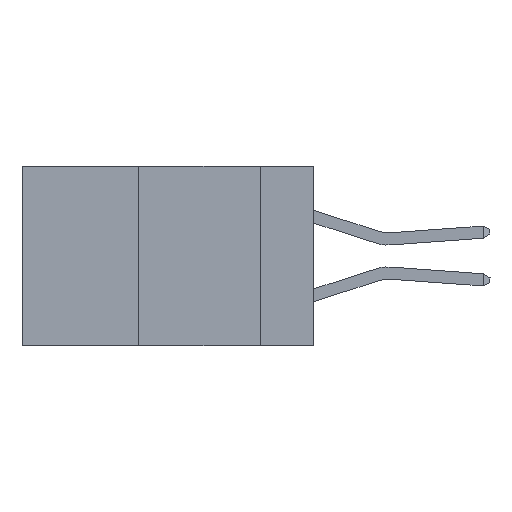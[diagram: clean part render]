
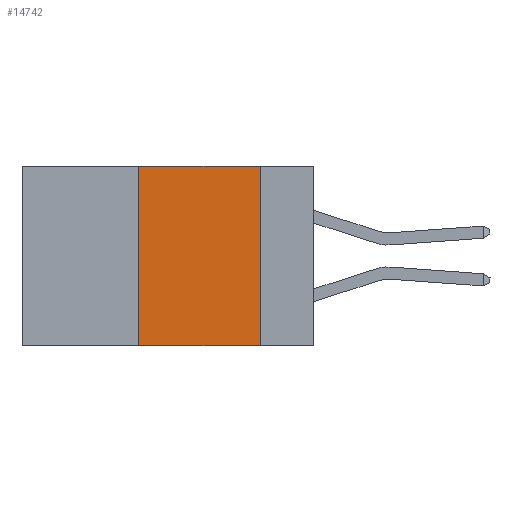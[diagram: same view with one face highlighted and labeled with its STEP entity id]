
A CAD part, left-side view. The second image highlights one B-rep face of the part: STEP entity #14742.
In plain terms, the highlighted planar face has unit normal (-1, 0, 0).
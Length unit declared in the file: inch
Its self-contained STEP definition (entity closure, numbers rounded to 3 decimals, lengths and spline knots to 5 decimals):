
#237 = CARTESIAN_POINT ( 'NONE',  ( 0., 0.11, 0. ) ) ;
#320 = EDGE_CURVE ( 'NONE', #1508, #4824, #4177, .T. ) ;
#327 = PLANE ( 'NONE',  #4135 ) ;
#705 = VECTOR ( 'NONE', #15442, 39.37008 ) ;
#934 = EDGE_CURVE ( 'NONE', #1508, #12777, #6030, .T. ) ;
#1080 = EDGE_CURVE ( 'NONE', #8344, #4824, #12422, .T. ) ;
#1280 = EDGE_CURVE ( 'NONE', #12777, #8344, #11835, .T. ) ;
#1335 = DIRECTION ( 'NONE',  ( 0., -1., 0. ) ) ;
#1414 = CARTESIAN_POINT ( 'NONE',  ( 0., 0.6, 0. ) ) ;
#1508 = VERTEX_POINT ( 'NONE', #4105 ) ;
#1845 = VECTOR ( 'NONE', #1335, 39.37008 ) ;
#3018 = CARTESIAN_POINT ( 'NONE',  ( 0., 0.6, -0.37 ) ) ;
#4105 = CARTESIAN_POINT ( 'NONE',  ( 0., 0.36, -0.37 ) ) ;
#4135 = AXIS2_PLACEMENT_3D ( 'NONE', #11725, #4278, #12941 ) ;
#4177 = LINE ( 'NONE', #3018, #705 ) ;
#4278 = DIRECTION ( 'NONE',  ( 1., 0., 0. ) ) ;
#4783 = ORIENTED_EDGE ( 'NONE', *, *, #934, .F. ) ;
#4824 = VERTEX_POINT ( 'NONE', #6636 ) ;
#5525 = CARTESIAN_POINT ( 'NONE',  ( 0., 0.36, 0. ) ) ;
#6030 = LINE ( 'NONE', #10517, #15502 ) ;
#6633 = FACE_OUTER_BOUND ( 'NONE', #8997, .T. ) ;
#6636 = CARTESIAN_POINT ( 'NONE',  ( 0., 0.11, -0.37 ) ) ;
#8344 = VERTEX_POINT ( 'NONE', #13882 ) ;
#8997 = EDGE_LOOP ( 'NONE', ( #9445, #13893, #4783, #11400 ) ) ;
#9445 = ORIENTED_EDGE ( 'NONE', *, *, #1080, .F. ) ;
#10517 = CARTESIAN_POINT ( 'NONE',  ( 0., 0.36, 0. ) ) ;
#11400 = ORIENTED_EDGE ( 'NONE', *, *, #320, .T. ) ;
#11469 = DIRECTION ( 'NONE',  ( 0., 0., 1. ) ) ;
#11725 = CARTESIAN_POINT ( 'NONE',  ( 0., 0.6, 0. ) ) ;
#11835 = LINE ( 'NONE', #1414, #1845 ) ;
#12422 = LINE ( 'NONE', #237, #16074 ) ;
#12777 = VERTEX_POINT ( 'NONE', #5525 ) ;
#12941 = DIRECTION ( 'NONE',  ( 0., 0., -1. ) ) ;
#13882 = CARTESIAN_POINT ( 'NONE',  ( 0., 0.11, 0. ) ) ;
#13893 = ORIENTED_EDGE ( 'NONE', *, *, #1280, .F. ) ;
#14742 = ADVANCED_FACE ( 'NONE', ( #6633 ), #327, .F. ) ;
#15442 = DIRECTION ( 'NONE',  ( 0., -1., 0. ) ) ;
#15502 = VECTOR ( 'NONE', #11469, 39.37008 ) ;
#15748 = DIRECTION ( 'NONE',  ( 0., 0., -1. ) ) ;
#16074 = VECTOR ( 'NONE', #15748, 39.37008 ) ;
